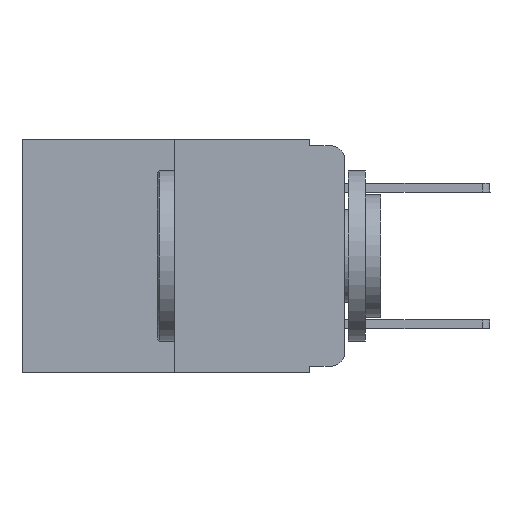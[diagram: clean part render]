
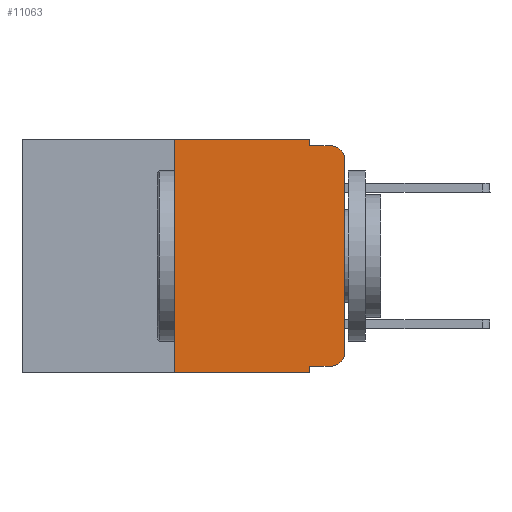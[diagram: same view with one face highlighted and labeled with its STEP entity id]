
A CAD part, left-side view. The second image highlights one B-rep face of the part: STEP entity #11063.
In plain terms, the highlighted planar face has unit normal (-1, 0, 0).
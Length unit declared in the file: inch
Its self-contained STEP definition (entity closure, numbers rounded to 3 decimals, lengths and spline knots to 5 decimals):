
#14 = CARTESIAN_POINT ( 'NONE',  ( 0., 0.02, -0.313 ) ) ;
#23 = VERTEX_POINT ( 'NONE', #8195 ) ;
#129 = EDGE_CURVE ( 'NONE', #9489, #11487, #337, .T. ) ;
#264 = VERTEX_POINT ( 'NONE', #5142 ) ;
#337 = LINE ( 'NONE', #5569, #4523 ) ;
#565 = CARTESIAN_POINT ( 'NONE',  ( 0., 0.051, -0.01 ) ) ;
#795 = DIRECTION ( 'NONE',  ( 0., -1., 0. ) ) ;
#883 = VERTEX_POINT ( 'NONE', #3004 ) ;
#1081 = VERTEX_POINT ( 'NONE', #2168 ) ;
#1144 = EDGE_CURVE ( 'NONE', #264, #9489, #6642, .T. ) ;
#1289 = DIRECTION ( 'NONE',  ( 0., 0., 1. ) ) ;
#1339 = DIRECTION ( 'NONE',  ( 0., -1., 0. ) ) ;
#1676 = ORIENTED_EDGE ( 'NONE', *, *, #5437, .T. ) ;
#1716 = CARTESIAN_POINT ( 'NONE',  ( 0., 0.051, 0. ) ) ;
#1875 = ORIENTED_EDGE ( 'NONE', *, *, #8704, .F. ) ;
#2149 = EDGE_CURVE ( 'NONE', #4172, #6814, #4535, .T. ) ;
#2168 = CARTESIAN_POINT ( 'NONE',  ( 0., 0.051, -0.01 ) ) ;
#2416 = ORIENTED_EDGE ( 'NONE', *, *, #1144, .F. ) ;
#2494 = DIRECTION ( 'NONE',  ( 0., 0., -1. ) ) ;
#2553 = AXIS2_PLACEMENT_3D ( 'NONE', #7532, #6729, #4009 ) ;
#2573 = VECTOR ( 'NONE', #795, 39.37008 ) ;
#2645 = LINE ( 'NONE', #6286, #9296 ) ;
#3004 = CARTESIAN_POINT ( 'NONE',  ( 0., 0.051, -0.333 ) ) ;
#3214 = PLANE ( 'NONE',  #5945 ) ;
#3272 = DIRECTION ( 'NONE',  ( 0., 0., -1. ) ) ;
#3482 = EDGE_CURVE ( 'NONE', #1081, #6340, #7843, .T. ) ;
#3597 = DIRECTION ( 'NONE',  ( 0., 0., 1. ) ) ;
#3683 = CIRCLE ( 'NONE', #6686, 0.02 ) ;
#3686 = CARTESIAN_POINT ( 'NONE',  ( 0., 0.473, -0.343 ) ) ;
#4009 = DIRECTION ( 'NONE',  ( 0., 0., -1. ) ) ;
#4094 = ORIENTED_EDGE ( 'NONE', *, *, #11518, .T. ) ;
#4120 = ORIENTED_EDGE ( 'NONE', *, *, #129, .F. ) ;
#4172 = VERTEX_POINT ( 'NONE', #8452 ) ;
#4278 = DIRECTION ( 'NONE',  ( 1., 0., 0. ) ) ;
#4293 = EDGE_LOOP ( 'NONE', ( #7992, #8153, #5379, #9712, #4120, #2416, #9405, #1875, #1676, #4094 ) ) ;
#4306 = DIRECTION ( 'NONE',  ( -1., 0., 0. ) ) ;
#4495 = EDGE_CURVE ( 'NONE', #11487, #1081, #2645, .T. ) ;
#4523 = VECTOR ( 'NONE', #8374, 39.37008 ) ;
#4535 = LINE ( 'NONE', #6204, #7972 ) ;
#4687 = VERTEX_POINT ( 'NONE', #5764 ) ;
#5142 = CARTESIAN_POINT ( 'NONE',  ( 0., 0.25, -0.343 ) ) ;
#5248 = DIRECTION ( 'NONE',  ( 0., 0., -1. ) ) ;
#5301 = VECTOR ( 'NONE', #1289, 39.37008 ) ;
#5379 = ORIENTED_EDGE ( 'NONE', *, *, #3482, .F. ) ;
#5437 = EDGE_CURVE ( 'NONE', #883, #4687, #11210, .T. ) ;
#5569 = CARTESIAN_POINT ( 'NONE',  ( 0., 0.473, 0. ) ) ;
#5604 = CARTESIAN_POINT ( 'NONE',  ( 0., 0.051, -0.333 ) ) ;
#5618 = CARTESIAN_POINT ( 'NONE',  ( 0., 0., -0.03 ) ) ;
#5764 = CARTESIAN_POINT ( 'NONE',  ( 0., 0.02, -0.333 ) ) ;
#5934 = CARTESIAN_POINT ( 'NONE',  ( 0., 0.473, 0. ) ) ;
#5945 = AXIS2_PLACEMENT_3D ( 'NONE', #5934, #4278, #3272 ) ;
#5947 = CARTESIAN_POINT ( 'NONE',  ( 0., 0.25, 0. ) ) ;
#6204 = CARTESIAN_POINT ( 'NONE',  ( 0., 0., 0. ) ) ;
#6235 = DIRECTION ( 'NONE',  ( 0., 0., -1. ) ) ;
#6244 = EDGE_CURVE ( 'NONE', #264, #23, #7148, .T. ) ;
#6286 = CARTESIAN_POINT ( 'NONE',  ( 0., 0.051, 0. ) ) ;
#6340 = VERTEX_POINT ( 'NONE', #9186 ) ;
#6642 = LINE ( 'NONE', #9333, #5301 ) ;
#6686 = AXIS2_PLACEMENT_3D ( 'NONE', #14, #4306, #5248 ) ;
#6729 = DIRECTION ( 'NONE',  ( -1., 0., 0. ) ) ;
#6814 = VERTEX_POINT ( 'NONE', #5618 ) ;
#7148 = LINE ( 'NONE', #3686, #7206 ) ;
#7206 = VECTOR ( 'NONE', #7841, 39.37008 ) ;
#7532 = CARTESIAN_POINT ( 'NONE',  ( 0., 0.02, -0.03 ) ) ;
#7841 = DIRECTION ( 'NONE',  ( 0., -1., 0. ) ) ;
#7843 = LINE ( 'NONE', #565, #2573 ) ;
#7931 = CARTESIAN_POINT ( 'NONE',  ( 0., 0.051, 0. ) ) ;
#7972 = VECTOR ( 'NONE', #3597, 39.37008 ) ;
#7992 = ORIENTED_EDGE ( 'NONE', *, *, #2149, .T. ) ;
#8153 = ORIENTED_EDGE ( 'NONE', *, *, #8469, .T. ) ;
#8195 = CARTESIAN_POINT ( 'NONE',  ( 0., 0.051, -0.343 ) ) ;
#8374 = DIRECTION ( 'NONE',  ( 0., -1., 0. ) ) ;
#8452 = CARTESIAN_POINT ( 'NONE',  ( 0., 0., -0.313 ) ) ;
#8469 = EDGE_CURVE ( 'NONE', #6814, #6340, #10766, .T. ) ;
#8704 = EDGE_CURVE ( 'NONE', #883, #23, #9765, .T. ) ;
#9186 = CARTESIAN_POINT ( 'NONE',  ( 0., 0.02, -0.01 ) ) ;
#9296 = VECTOR ( 'NONE', #6235, 39.37008 ) ;
#9333 = CARTESIAN_POINT ( 'NONE',  ( 0., 0.25, 0. ) ) ;
#9405 = ORIENTED_EDGE ( 'NONE', *, *, #6244, .T. ) ;
#9489 = VERTEX_POINT ( 'NONE', #5947 ) ;
#9658 = VECTOR ( 'NONE', #2494, 39.37008 ) ;
#9712 = ORIENTED_EDGE ( 'NONE', *, *, #4495, .F. ) ;
#9765 = LINE ( 'NONE', #1716, #9658 ) ;
#10355 = FACE_OUTER_BOUND ( 'NONE', #4293, .T. ) ;
#10733 = VECTOR ( 'NONE', #1339, 39.37008 ) ;
#10766 = CIRCLE ( 'NONE', #2553, 0.02 ) ;
#11063 = ADVANCED_FACE ( 'NONE', ( #10355 ), #3214, .F. ) ;
#11210 = LINE ( 'NONE', #5604, #10733 ) ;
#11487 = VERTEX_POINT ( 'NONE', #7931 ) ;
#11518 = EDGE_CURVE ( 'NONE', #4687, #4172, #3683, .T. ) ;
